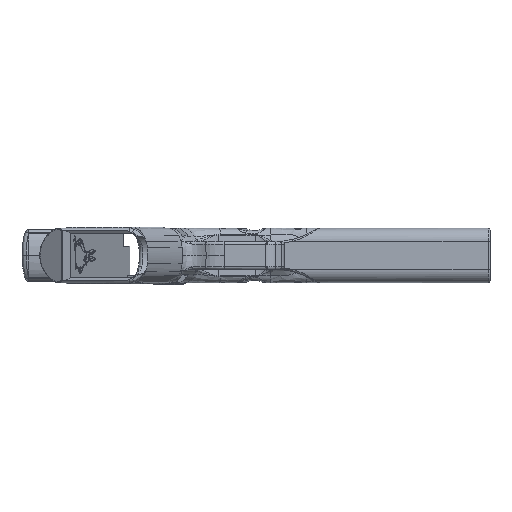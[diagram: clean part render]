
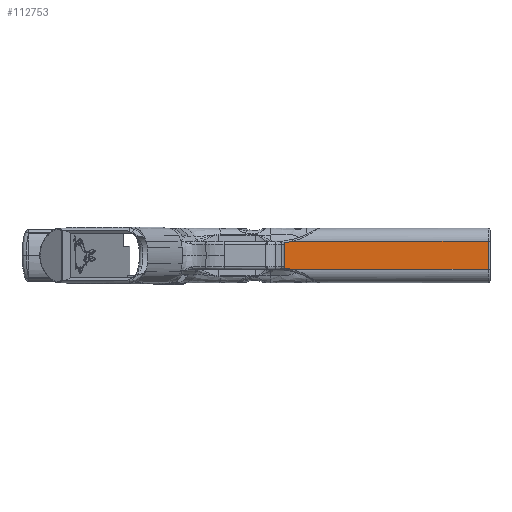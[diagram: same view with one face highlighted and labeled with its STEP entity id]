
A CAD part, front view. The second image highlights one B-rep face of the part: STEP entity #112753.
In plain terms, the highlighted planar face has unit normal (0, -1, 0).
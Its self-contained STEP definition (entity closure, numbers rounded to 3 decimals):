
#12302=B_SPLINE_CURVE_WITH_KNOTS('',3,(#136484,#136485,#136486,#136487),
 .UNSPECIFIED.,.F.,.F.,(4,4),(1.226,1.702),
 .UNSPECIFIED.);
#12303=B_SPLINE_CURVE_WITH_KNOTS('',3,(#136491,#136492,#136493,#136494),
 .UNSPECIFIED.,.F.,.F.,(4,4),(0.311,0.807),
 .UNSPECIFIED.);
#12304=B_SPLINE_CURVE_WITH_KNOTS('',3,(#136496,#136497,#136498,#136499,
#136500,#136501),.UNSPECIFIED.,.F.,.F.,(4,2,4),(-0.963,-0.939,
-0.935),.UNSPECIFIED.);
#13295=PLANE('',#119189);
#15252=FACE_OUTER_BOUND('',#21652,.T.);
#21652=EDGE_LOOP('',(#76588,#76589,#76590,#76591,#76592,#76593,#76594,#76595,
#76596,#76597));
#28317=LINE('',#136249,#37192);
#28355=LINE('',#136455,#37230);
#28357=LINE('',#136479,#37232);
#28358=LINE('',#136481,#37233);
#28359=LINE('',#136483,#37234);
#28360=LINE('',#136489,#37235);
#28361=LINE('',#136502,#37236);
#37192=VECTOR('',#121910,10.);
#37230=VECTOR('',#121996,10.);
#37232=VECTOR('',#122000,10.);
#37233=VECTOR('',#122001,10.);
#37234=VECTOR('',#122002,10.);
#37235=VECTOR('',#122003,10.);
#37236=VECTOR('',#122004,10.);
#46544=VERTEX_POINT('',#136241);
#46546=VERTEX_POINT('',#136247);
#46602=VERTEX_POINT('',#136454);
#46606=VERTEX_POINT('',#136477);
#46607=VERTEX_POINT('',#136478);
#46608=VERTEX_POINT('',#136480);
#46609=VERTEX_POINT('',#136482);
#46610=VERTEX_POINT('',#136488);
#46611=VERTEX_POINT('',#136490);
#46612=VERTEX_POINT('',#136495);
#58449=EDGE_CURVE('',#46546,#46544,#28317,.T.);
#58514=EDGE_CURVE('',#46602,#46544,#28355,.F.);
#58519=EDGE_CURVE('',#46606,#46607,#28357,.T.);
#58520=EDGE_CURVE('',#46608,#46606,#28358,.T.);
#58521=EDGE_CURVE('',#46609,#46608,#28359,.F.);
#58522=EDGE_CURVE('',#46602,#46609,#12302,.T.);
#58523=EDGE_CURVE('',#46610,#46546,#28360,.T.);
#58524=EDGE_CURVE('',#46611,#46610,#12303,.T.);
#58525=EDGE_CURVE('',#46612,#46611,#12304,.T.);
#58526=EDGE_CURVE('',#46607,#46612,#28361,.T.);
#76588=ORIENTED_EDGE('',*,*,#58519,.F.);
#76589=ORIENTED_EDGE('',*,*,#58520,.F.);
#76590=ORIENTED_EDGE('',*,*,#58521,.F.);
#76591=ORIENTED_EDGE('',*,*,#58522,.F.);
#76592=ORIENTED_EDGE('',*,*,#58514,.T.);
#76593=ORIENTED_EDGE('',*,*,#58449,.F.);
#76594=ORIENTED_EDGE('',*,*,#58523,.F.);
#76595=ORIENTED_EDGE('',*,*,#58524,.F.);
#76596=ORIENTED_EDGE('',*,*,#58525,.F.);
#76597=ORIENTED_EDGE('',*,*,#58526,.F.);
#112753=ADVANCED_FACE('',(#15252),#13295,.T.);
#119189=AXIS2_PLACEMENT_3D('',#136476,#121998,#121999);
#121910=DIRECTION('',(0.,0.,-1.));
#121996=DIRECTION('',(-1.,0.,0.));
#121998=DIRECTION('center_axis',(0.,-1.,0.));
#121999=DIRECTION('ref_axis',(0.,0.,1.));
#122000=DIRECTION('',(0.,0.,1.));
#122001=DIRECTION('',(1.,0.,0.));
#122002=DIRECTION('',(0.,0.,-1.));
#122003=DIRECTION('',(1.,0.,0.));
#122004=DIRECTION('',(0.,0.,1.));
#136241=CARTESIAN_POINT('',(122.908,-29.675,-7.4));
#136247=CARTESIAN_POINT('',(122.908,-29.675,7.4));
#136249=CARTESIAN_POINT('',(122.908,-29.675,-7.2));
#136454=CARTESIAN_POINT('',(19.618,-29.675,-7.4));
#136455=CARTESIAN_POINT('',(11.959,-29.675,-7.4));
#136476=CARTESIAN_POINT('Origin',(123.918,-29.675,-14.4));
#136477=CARTESIAN_POINT('',(14.923,-29.675,-6.));
#136478=CARTESIAN_POINT('',(14.923,-29.675,5.9));
#136479=CARTESIAN_POINT('',(14.923,-29.675,-7.225));
#136480=CARTESIAN_POINT('',(14.923,-29.675,-6.));
#136481=CARTESIAN_POINT('',(69.443,-29.675,-6.));
#136482=CARTESIAN_POINT('',(14.923,-29.675,-6.598));
#136483=CARTESIAN_POINT('',(14.923,-29.675,-7.225));
#136484=CARTESIAN_POINT('Ctrl Pts',(19.618,-29.675,-7.4));
#136485=CARTESIAN_POINT('Ctrl Pts',(18.074,-29.675,
-7.032));
#136486=CARTESIAN_POINT('Ctrl Pts',(16.502,-29.675,
-6.764));
#136487=CARTESIAN_POINT('Ctrl Pts',(14.923,-29.675,
-6.598));
#136488=CARTESIAN_POINT('',(19.672,-29.675,7.4));
#136489=CARTESIAN_POINT('',(11.959,-29.675,7.4));
#136490=CARTESIAN_POINT('',(14.774,-29.675,6.578));
#136491=CARTESIAN_POINT('Ctrl Pts',(14.774,-29.675,
6.578));
#136492=CARTESIAN_POINT('Ctrl Pts',(16.423,-29.675,
6.743));
#136493=CARTESIAN_POINT('Ctrl Pts',(18.064,-29.675,
7.017));
#136494=CARTESIAN_POINT('Ctrl Pts',(19.672,-29.675,
7.4));
#136495=CARTESIAN_POINT('',(14.923,-29.675,6.085));
#136496=CARTESIAN_POINT('Ctrl Pts',(14.923,-29.675,
6.085));
#136497=CARTESIAN_POINT('Ctrl Pts',(14.905,-29.675,
6.231));
#136498=CARTESIAN_POINT('Ctrl Pts',(14.866,-29.675,
6.373));
#136499=CARTESIAN_POINT('Ctrl Pts',(14.796,-29.675,
6.532));
#136500=CARTESIAN_POINT('Ctrl Pts',(14.785,-29.675,
6.555));
#136501=CARTESIAN_POINT('Ctrl Pts',(14.774,-29.675,
6.578));
#136502=CARTESIAN_POINT('',(14.923,-29.675,-10.9));
